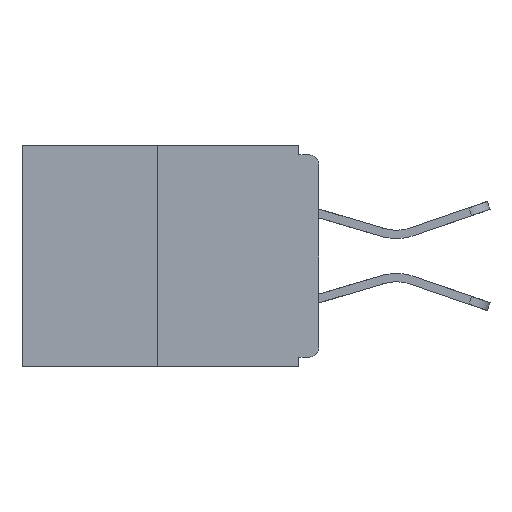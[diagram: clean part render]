
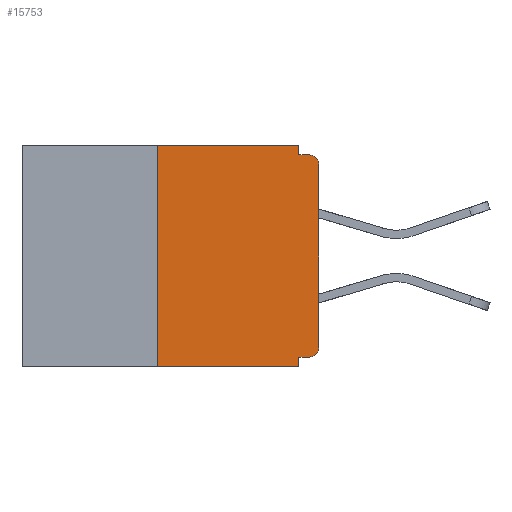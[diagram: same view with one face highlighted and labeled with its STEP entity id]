
A CAD part, left-side view. The second image highlights one B-rep face of the part: STEP entity #15753.
In plain terms, the highlighted planar face has unit normal (-1, 0, 0).
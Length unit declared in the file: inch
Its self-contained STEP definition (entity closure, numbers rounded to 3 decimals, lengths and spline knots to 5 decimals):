
#248 = VECTOR ( 'NONE', #6483, 39.37008 ) ;
#404 = EDGE_LOOP ( 'NONE', ( #15835, #15229, #18162, #17763, #5657, #24936, #5414, #1329, #18819, #15251 ) ) ;
#1313 = DIRECTION ( 'NONE',  ( 0., 0., -1. ) ) ;
#1329 = ORIENTED_EDGE ( 'NONE', *, *, #30068, .T. ) ;
#1728 = EDGE_CURVE ( 'NONE', #29160, #19971, #19824, .T. ) ;
#2026 = CARTESIAN_POINT ( 'NONE',  ( 0., 0.46, -0.343 ) ) ;
#2092 = LINE ( 'NONE', #2771, #27209 ) ;
#2771 = CARTESIAN_POINT ( 'NONE',  ( 0., 0.031, 0. ) ) ;
#2877 = VERTEX_POINT ( 'NONE', #24443 ) ;
#3026 = CARTESIAN_POINT ( 'NONE',  ( 0., 0.031, -0.015 ) ) ;
#3042 = EDGE_CURVE ( 'NONE', #16873, #29160, #19920, .T. ) ;
#3098 = AXIS2_PLACEMENT_3D ( 'NONE', #10879, #16009, #1313 ) ;
#3597 = CARTESIAN_POINT ( 'NONE',  ( 0., 0.46, 0. ) ) ;
#4097 = LINE ( 'NONE', #5696, #29570 ) ;
#4164 = FACE_OUTER_BOUND ( 'NONE', #404, .T. ) ;
#4322 = CARTESIAN_POINT ( 'NONE',  ( 0., 0.031, -0.343 ) ) ;
#4571 = LINE ( 'NONE', #2026, #30041 ) ;
#5109 = AXIS2_PLACEMENT_3D ( 'NONE', #22399, #12635, #27481 ) ;
#5177 = LINE ( 'NONE', #13628, #28352 ) ;
#5414 = ORIENTED_EDGE ( 'NONE', *, *, #1728, .T. ) ;
#5441 = AXIS2_PLACEMENT_3D ( 'NONE', #3597, #8658, #23368 ) ;
#5657 = ORIENTED_EDGE ( 'NONE', *, *, #8203, .F. ) ;
#5696 = CARTESIAN_POINT ( 'NONE',  ( 0., 0., -0.328 ) ) ;
#6468 = CARTESIAN_POINT ( 'NONE',  ( 0., 0.25, -0.343 ) ) ;
#6483 = DIRECTION ( 'NONE',  ( 0., 0., -1. ) ) ;
#7468 = EDGE_CURVE ( 'NONE', #28135, #2877, #31529, .T. ) ;
#7801 = VECTOR ( 'NONE', #25181, 39.37008 ) ;
#7888 = EDGE_CURVE ( 'NONE', #9355, #20332, #14170, .T. ) ;
#8203 = EDGE_CURVE ( 'NONE', #16873, #13310, #4097, .T. ) ;
#8658 = DIRECTION ( 'NONE',  ( 1., 0., 0. ) ) ;
#9160 = EDGE_CURVE ( 'NONE', #12580, #30659, #4571, .T. ) ;
#9355 = VERTEX_POINT ( 'NONE', #25365 ) ;
#10677 = VECTOR ( 'NONE', #23476, 39.37008 ) ;
#10879 = CARTESIAN_POINT ( 'NONE',  ( 0., 0.015, -0.313 ) ) ;
#11001 = CARTESIAN_POINT ( 'NONE',  ( 0., 0.46, 0. ) ) ;
#12033 = DIRECTION ( 'NONE',  ( 0., -1., 0. ) ) ;
#12580 = VERTEX_POINT ( 'NONE', #6468 ) ;
#12635 = DIRECTION ( 'NONE',  ( -1., 0., 0. ) ) ;
#12638 = VECTOR ( 'NONE', #15636, 39.37008 ) ;
#12971 = LINE ( 'NONE', #4322, #248 ) ;
#13310 = VERTEX_POINT ( 'NONE', #23550 ) ;
#13628 = CARTESIAN_POINT ( 'NONE',  ( 0., 0.25, 0. ) ) ;
#14170 = LINE ( 'NONE', #11001, #10677 ) ;
#15229 = ORIENTED_EDGE ( 'NONE', *, *, #29924, .F. ) ;
#15251 = ORIENTED_EDGE ( 'NONE', *, *, #17458, .F. ) ;
#15636 = DIRECTION ( 'NONE',  ( 0., -1., 0. ) ) ;
#15753 = ADVANCED_FACE ( 'NONE', ( #4164 ), #25758, .F. ) ;
#15835 = ORIENTED_EDGE ( 'NONE', *, *, #7888, .F. ) ;
#16009 = DIRECTION ( 'NONE',  ( -1., 0., 0. ) ) ;
#16263 = DIRECTION ( 'NONE',  ( 0., 1., 0. ) ) ;
#16746 = CARTESIAN_POINT ( 'NONE',  ( 0., 0., 0. ) ) ;
#16873 = VERTEX_POINT ( 'NONE', #25866 ) ;
#17458 = EDGE_CURVE ( 'NONE', #20332, #28135, #2092, .T. ) ;
#17763 = ORIENTED_EDGE ( 'NONE', *, *, #28749, .F. ) ;
#18162 = ORIENTED_EDGE ( 'NONE', *, *, #9160, .T. ) ;
#18819 = ORIENTED_EDGE ( 'NONE', *, *, #7468, .F. ) ;
#19824 = LINE ( 'NONE', #16746, #7801 ) ;
#19920 = CIRCLE ( 'NONE', #3098, 0.015 ) ;
#19971 = VERTEX_POINT ( 'NONE', #20192 ) ;
#20077 = DIRECTION ( 'NONE',  ( 0., 0., -1. ) ) ;
#20192 = CARTESIAN_POINT ( 'NONE',  ( 0., 0., -0.03 ) ) ;
#20332 = VERTEX_POINT ( 'NONE', #20446 ) ;
#20446 = CARTESIAN_POINT ( 'NONE',  ( 0., 0.031, 0. ) ) ;
#22399 = CARTESIAN_POINT ( 'NONE',  ( 0., 0.015, -0.03 ) ) ;
#23368 = DIRECTION ( 'NONE',  ( 0., 0., -1. ) ) ;
#23476 = DIRECTION ( 'NONE',  ( 0., -1., 0. ) ) ;
#23550 = CARTESIAN_POINT ( 'NONE',  ( 0., 0.031, -0.328 ) ) ;
#24443 = CARTESIAN_POINT ( 'NONE',  ( 0., 0.015, -0.015 ) ) ;
#24936 = ORIENTED_EDGE ( 'NONE', *, *, #3042, .T. ) ;
#25181 = DIRECTION ( 'NONE',  ( 0., 0., 1. ) ) ;
#25342 = CARTESIAN_POINT ( 'NONE',  ( 0., 0.031, -0.343 ) ) ;
#25365 = CARTESIAN_POINT ( 'NONE',  ( 0., 0.25, 0. ) ) ;
#25758 = PLANE ( 'NONE',  #5441 ) ;
#25866 = CARTESIAN_POINT ( 'NONE',  ( 0., 0.015, -0.328 ) ) ;
#26297 = DIRECTION ( 'NONE',  ( 0., 0., 1. ) ) ;
#27209 = VECTOR ( 'NONE', #20077, 39.37008 ) ;
#27481 = DIRECTION ( 'NONE',  ( 0., 0., -1. ) ) ;
#27957 = CARTESIAN_POINT ( 'NONE',  ( 0., 0., -0.015 ) ) ;
#28135 = VERTEX_POINT ( 'NONE', #3026 ) ;
#28352 = VECTOR ( 'NONE', #26297, 39.37008 ) ;
#28749 = EDGE_CURVE ( 'NONE', #13310, #30659, #12971, .T. ) ;
#29160 = VERTEX_POINT ( 'NONE', #30779 ) ;
#29570 = VECTOR ( 'NONE', #16263, 39.37008 ) ;
#29924 = EDGE_CURVE ( 'NONE', #12580, #9355, #5177, .T. ) ;
#30041 = VECTOR ( 'NONE', #12033, 39.37008 ) ;
#30068 = EDGE_CURVE ( 'NONE', #19971, #2877, #30599, .T. ) ;
#30599 = CIRCLE ( 'NONE', #5109, 0.015 ) ;
#30659 = VERTEX_POINT ( 'NONE', #25342 ) ;
#30779 = CARTESIAN_POINT ( 'NONE',  ( 0., 0., -0.313 ) ) ;
#31529 = LINE ( 'NONE', #27957, #12638 ) ;
